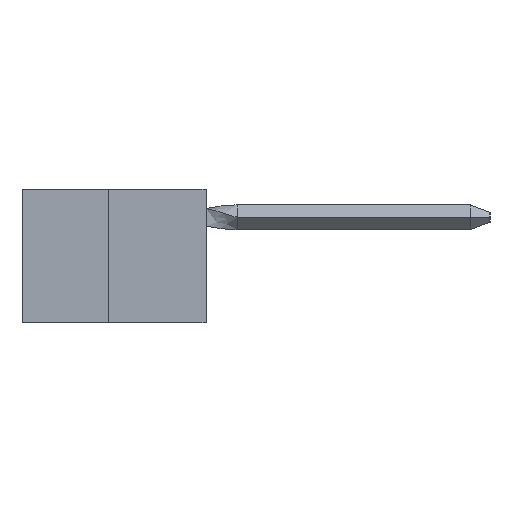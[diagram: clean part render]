
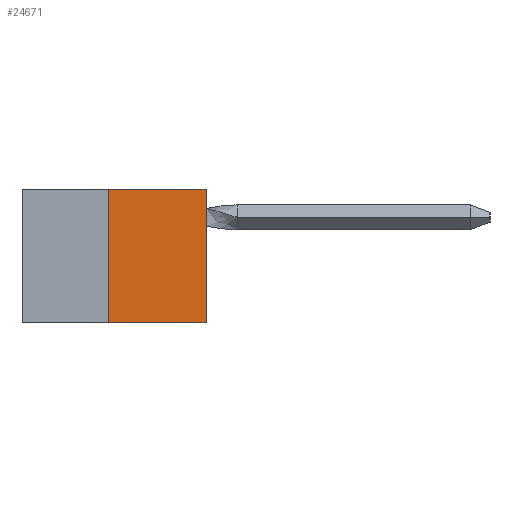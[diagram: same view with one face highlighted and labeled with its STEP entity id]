
A CAD part, left-side view. The second image highlights one B-rep face of the part: STEP entity #24671.
In plain terms, the highlighted planar face has unit normal (-1, 0, 0).
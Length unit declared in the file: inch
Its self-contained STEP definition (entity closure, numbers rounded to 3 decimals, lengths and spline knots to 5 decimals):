
#522 = AXIS2_PLACEMENT_3D ( 'NONE', #11684, #29166, #25463 ) ;
#3548 = LINE ( 'NONE', #44202, #41461 ) ;
#5618 = ORIENTED_EDGE ( 'NONE', *, *, #22801, .T. ) ;
#6408 = EDGE_CURVE ( 'NONE', #41619, #19554, #3548, .T. ) ;
#6686 = DIRECTION ( 'NONE',  ( 0., 0., 1. ) ) ;
#7803 = DIRECTION ( 'NONE',  ( 0., -1., 0. ) ) ;
#11684 = CARTESIAN_POINT ( 'NONE',  ( 0., 0.473, 0. ) ) ;
#13079 = CARTESIAN_POINT ( 'NONE',  ( 0., 0.25, -0.343 ) ) ;
#13732 = CARTESIAN_POINT ( 'NONE',  ( 0., 0.473, -0.343 ) ) ;
#13995 = VERTEX_POINT ( 'NONE', #13079 ) ;
#15933 = LINE ( 'NONE', #21682, #37850 ) ;
#18372 = VECTOR ( 'NONE', #26184, 39.37008 ) ;
#19554 = VERTEX_POINT ( 'NONE', #23706 ) ;
#20470 = FACE_OUTER_BOUND ( 'NONE', #32289, .T. ) ;
#21682 = CARTESIAN_POINT ( 'NONE',  ( 0., 0.473, 0. ) ) ;
#22801 = EDGE_CURVE ( 'NONE', #13995, #41619, #30685, .T. ) ;
#23706 = CARTESIAN_POINT ( 'NONE',  ( 0., 0., 0. ) ) ;
#24671 = ADVANCED_FACE ( 'NONE', ( #20470 ), #38298, .F. ) ;
#25463 = DIRECTION ( 'NONE',  ( 0., 0., -1. ) ) ;
#26184 = DIRECTION ( 'NONE',  ( 0., 0., 1. ) ) ;
#27038 = ORIENTED_EDGE ( 'NONE', *, *, #6408, .T. ) ;
#28526 = LINE ( 'NONE', #43196, #18372 ) ;
#29137 = VECTOR ( 'NONE', #33926, 39.37008 ) ;
#29166 = DIRECTION ( 'NONE',  ( 1., 0., 0. ) ) ;
#29813 = ORIENTED_EDGE ( 'NONE', *, *, #32647, .F. ) ;
#30685 = LINE ( 'NONE', #13732, #29137 ) ;
#32289 = EDGE_LOOP ( 'NONE', ( #29813, #35715, #5618, #27038 ) ) ;
#32647 = EDGE_CURVE ( 'NONE', #34115, #19554, #15933, .T. ) ;
#33926 = DIRECTION ( 'NONE',  ( 0., -1., 0. ) ) ;
#34115 = VERTEX_POINT ( 'NONE', #40063 ) ;
#34172 = CARTESIAN_POINT ( 'NONE',  ( 0., 0., -0.343 ) ) ;
#35715 = ORIENTED_EDGE ( 'NONE', *, *, #37426, .F. ) ;
#37426 = EDGE_CURVE ( 'NONE', #13995, #34115, #28526, .T. ) ;
#37850 = VECTOR ( 'NONE', #7803, 39.37008 ) ;
#38298 = PLANE ( 'NONE',  #522 ) ;
#40063 = CARTESIAN_POINT ( 'NONE',  ( 0., 0.25, 0. ) ) ;
#41461 = VECTOR ( 'NONE', #6686, 39.37008 ) ;
#41619 = VERTEX_POINT ( 'NONE', #34172 ) ;
#43196 = CARTESIAN_POINT ( 'NONE',  ( 0., 0.25, 0. ) ) ;
#44202 = CARTESIAN_POINT ( 'NONE',  ( 0., 0., 0. ) ) ;
